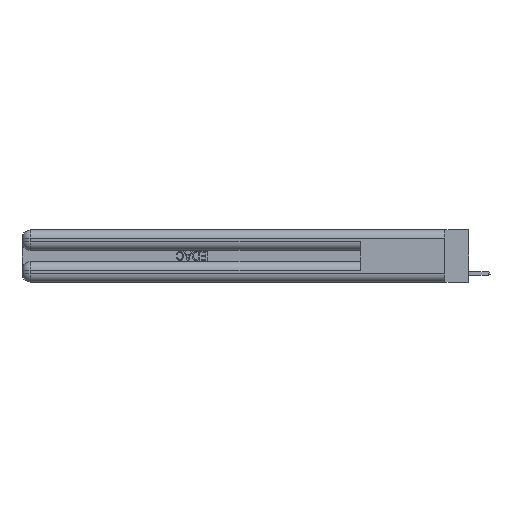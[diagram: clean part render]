
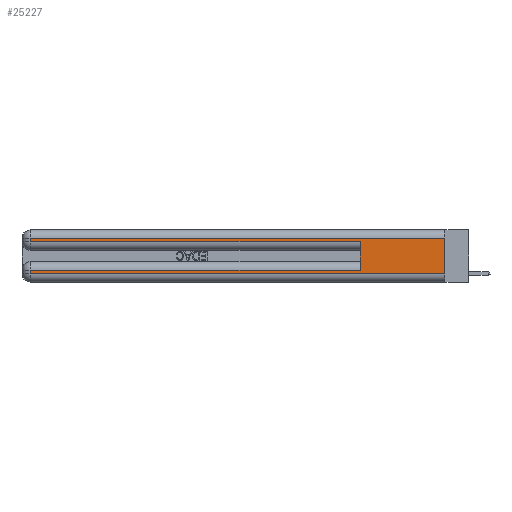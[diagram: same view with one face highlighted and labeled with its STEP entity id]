
A CAD part, left-side view. The second image highlights one B-rep face of the part: STEP entity #25227.
In plain terms, the highlighted planar face has unit normal (-1, 0, 0).
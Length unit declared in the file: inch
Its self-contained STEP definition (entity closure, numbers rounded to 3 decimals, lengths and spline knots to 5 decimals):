
#45 = CARTESIAN_POINT ( 'NONE',  ( 0., 0., 0.37 ) ) ;
#982 = EDGE_LOOP ( 'NONE', ( #19356, #27275, #20736, #12216, #11413, #15934, #15282, #5406 ) ) ;
#3345 = DIRECTION ( 'NONE',  ( 1., 0., 0. ) ) ;
#3597 = LINE ( 'NONE', #23945, #17672 ) ;
#4072 = DIRECTION ( 'NONE',  ( 0., 0., -1. ) ) ;
#4158 = CARTESIAN_POINT ( 'NONE',  ( 0., 2.94, 0.085 ) ) ;
#4567 = VECTOR ( 'NONE', #7463, 39.37008 ) ;
#5123 = VERTEX_POINT ( 'NONE', #21376 ) ;
#5406 = ORIENTED_EDGE ( 'NONE', *, *, #17136, .T. ) ;
#5924 = EDGE_CURVE ( 'NONE', #5123, #26729, #12114, .T. ) ;
#6009 = AXIS2_PLACEMENT_3D ( 'NONE', #14507, #3345, #4072 ) ;
#6836 = EDGE_CURVE ( 'NONE', #18628, #22932, #27337, .T. ) ;
#6942 = EDGE_CURVE ( 'NONE', #23817, #26729, #3597, .T. ) ;
#6980 = VECTOR ( 'NONE', #17937, 39.37008 ) ;
#7411 = CARTESIAN_POINT ( 'NONE',  ( 0., 0.6, 0.145 ) ) ;
#7463 = DIRECTION ( 'NONE',  ( 0., 1., 0. ) ) ;
#7727 = FACE_OUTER_BOUND ( 'NONE', #982, .T. ) ;
#7928 = DIRECTION ( 'NONE',  ( 0., -1., 0. ) ) ;
#8683 = VECTOR ( 'NONE', #21027, 39.37008 ) ;
#10091 = DIRECTION ( 'NONE',  ( 0., 0., -1. ) ) ;
#10491 = DIRECTION ( 'NONE',  ( 0., -1., 0. ) ) ;
#11413 = ORIENTED_EDGE ( 'NONE', *, *, #5924, .F. ) ;
#11866 = VERTEX_POINT ( 'NONE', #4158 ) ;
#12048 = CARTESIAN_POINT ( 'NONE',  ( 0., 2.94, 0.285 ) ) ;
#12114 = LINE ( 'NONE', #7411, #8683 ) ;
#12162 = LINE ( 'NONE', #27528, #4567 ) ;
#12216 = ORIENTED_EDGE ( 'NONE', *, *, #6942, .T. ) ;
#12310 = EDGE_CURVE ( 'NONE', #11866, #17727, #25321, .T. ) ;
#13882 = CARTESIAN_POINT ( 'NONE',  ( 0., 0., 0.31 ) ) ;
#14507 = CARTESIAN_POINT ( 'NONE',  ( 0., 0., 0.37 ) ) ;
#14573 = VERTEX_POINT ( 'NONE', #23696 ) ;
#14597 = CARTESIAN_POINT ( 'NONE',  ( 0., 2.94, 0.06 ) ) ;
#15282 = ORIENTED_EDGE ( 'NONE', *, *, #12310, .T. ) ;
#15934 = ORIENTED_EDGE ( 'NONE', *, *, #24074, .T. ) ;
#16178 = VECTOR ( 'NONE', #28317, 39.37008 ) ;
#16260 = DIRECTION ( 'NONE',  ( 0., 1., 0. ) ) ;
#16691 = PLANE ( 'NONE',  #6009 ) ;
#17136 = EDGE_CURVE ( 'NONE', #17727, #14573, #19076, .T. ) ;
#17672 = VECTOR ( 'NONE', #10491, 39.37008 ) ;
#17727 = VERTEX_POINT ( 'NONE', #14597 ) ;
#17937 = DIRECTION ( 'NONE',  ( 0., 0., -1. ) ) ;
#18628 = VERTEX_POINT ( 'NONE', #13882 ) ;
#19076 = LINE ( 'NONE', #26222, #24427 ) ;
#19356 = ORIENTED_EDGE ( 'NONE', *, *, #28600, .F. ) ;
#19428 = CARTESIAN_POINT ( 'NONE',  ( 0., 2.94, 0.37 ) ) ;
#20327 = CARTESIAN_POINT ( 'NONE',  ( 0., 2.94, 0.31 ) ) ;
#20736 = ORIENTED_EDGE ( 'NONE', *, *, #20989, .T. ) ;
#20989 = EDGE_CURVE ( 'NONE', #22932, #23817, #21591, .T. ) ;
#21027 = DIRECTION ( 'NONE',  ( 0., 0., 1. ) ) ;
#21376 = CARTESIAN_POINT ( 'NONE',  ( 0., 0.6, 0.085 ) ) ;
#21591 = LINE ( 'NONE', #19428, #16178 ) ;
#22415 = CARTESIAN_POINT ( 'NONE',  ( 0., 2.94, 0.37 ) ) ;
#22932 = VERTEX_POINT ( 'NONE', #20327 ) ;
#23237 = CARTESIAN_POINT ( 'NONE',  ( 0., 0., 0.31 ) ) ;
#23696 = CARTESIAN_POINT ( 'NONE',  ( 0., 0., 0.06 ) ) ;
#23817 = VERTEX_POINT ( 'NONE', #12048 ) ;
#23945 = CARTESIAN_POINT ( 'NONE',  ( 0., 0., 0.285 ) ) ;
#24074 = EDGE_CURVE ( 'NONE', #5123, #11866, #12162, .T. ) ;
#24427 = VECTOR ( 'NONE', #7928, 39.37008 ) ;
#25040 = LINE ( 'NONE', #45, #6980 ) ;
#25227 = ADVANCED_FACE ( 'NONE', ( #7727 ), #16691, .F. ) ;
#25321 = LINE ( 'NONE', #22415, #26685 ) ;
#26222 = CARTESIAN_POINT ( 'NONE',  ( 0., 0., 0.06 ) ) ;
#26685 = VECTOR ( 'NONE', #10091, 39.37008 ) ;
#26729 = VERTEX_POINT ( 'NONE', #27958 ) ;
#27275 = ORIENTED_EDGE ( 'NONE', *, *, #6836, .T. ) ;
#27337 = LINE ( 'NONE', #23237, #28343 ) ;
#27528 = CARTESIAN_POINT ( 'NONE',  ( 0., 0., 0.085 ) ) ;
#27958 = CARTESIAN_POINT ( 'NONE',  ( 0., 0.6, 0.285 ) ) ;
#28317 = DIRECTION ( 'NONE',  ( 0., 0., -1. ) ) ;
#28343 = VECTOR ( 'NONE', #16260, 39.37008 ) ;
#28600 = EDGE_CURVE ( 'NONE', #18628, #14573, #25040, .T. ) ;
